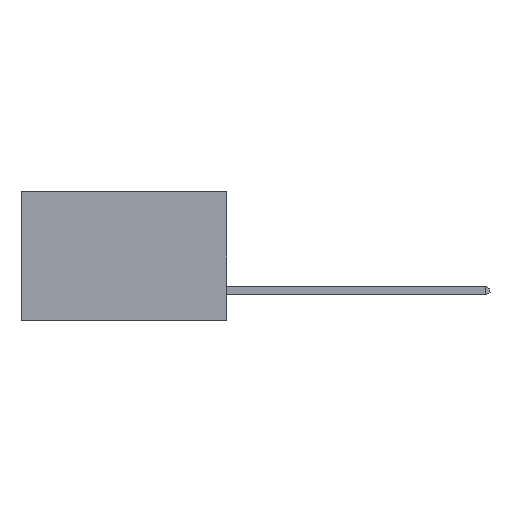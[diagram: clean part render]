
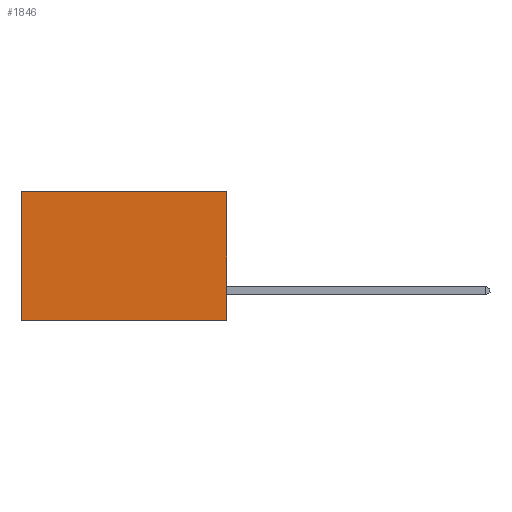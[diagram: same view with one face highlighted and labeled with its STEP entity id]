
A CAD part, left-side view. The second image highlights one B-rep face of the part: STEP entity #1846.
In plain terms, the highlighted planar face has unit normal (-1, 0, 0).
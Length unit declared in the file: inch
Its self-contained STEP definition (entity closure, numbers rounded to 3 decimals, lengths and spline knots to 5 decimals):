
#250 = CARTESIAN_POINT ( 'NONE',  ( 0.277, 0., -0.37 ) ) ;
#343 = DIRECTION ( 'NONE',  ( 1., 0., 0. ) ) ;
#647 = VECTOR ( 'NONE', #4072, 39.37008 ) ;
#1846 = ADVANCED_FACE ( 'NONE', ( #2296 ), #9590, .F. ) ;
#1884 = ORIENTED_EDGE ( 'NONE', *, *, #5309, .T. ) ;
#1910 = ORIENTED_EDGE ( 'NONE', *, *, #5973, .F. ) ;
#1949 = ORIENTED_EDGE ( 'NONE', *, *, #6731, .F. ) ;
#1982 = CARTESIAN_POINT ( 'NONE',  ( 0.277, 0.59, -0.37 ) ) ;
#2050 = ORIENTED_EDGE ( 'NONE', *, *, #12123, .T. ) ;
#2061 = DIRECTION ( 'NONE',  ( 0., 0., -1. ) ) ;
#2296 = FACE_OUTER_BOUND ( 'NONE', #9762, .T. ) ;
#2571 = VECTOR ( 'NONE', #3157, 39.37008 ) ;
#2828 = VERTEX_POINT ( 'NONE', #1982 ) ;
#3022 = CARTESIAN_POINT ( 'NONE',  ( 0.277, 0., 0. ) ) ;
#3157 = DIRECTION ( 'NONE',  ( 0., 0., -1. ) ) ;
#4072 = DIRECTION ( 'NONE',  ( 0., 1., 0. ) ) ;
#5309 = EDGE_CURVE ( 'NONE', #9479, #2828, #12591, .T. ) ;
#5416 = VECTOR ( 'NONE', #11059, 39.37008 ) ;
#5551 = VECTOR ( 'NONE', #2061, 39.37008 ) ;
#5873 = LINE ( 'NONE', #7092, #5551 ) ;
#5973 = EDGE_CURVE ( 'NONE', #10830, #2828, #7963, .T. ) ;
#6114 = LINE ( 'NONE', #3022, #647 ) ;
#6232 = CARTESIAN_POINT ( 'NONE',  ( 0.277, 0., -0.37 ) ) ;
#6429 = VERTEX_POINT ( 'NONE', #9653 ) ;
#6731 = EDGE_CURVE ( 'NONE', #6429, #10830, #5873, .T. ) ;
#7092 = CARTESIAN_POINT ( 'NONE',  ( 0.277, 0., -0.37 ) ) ;
#7963 = LINE ( 'NONE', #9150, #5416 ) ;
#9150 = CARTESIAN_POINT ( 'NONE',  ( 0.277, 0., -0.37 ) ) ;
#9152 = AXIS2_PLACEMENT_3D ( 'NONE', #6232, #343, #9777 ) ;
#9458 = CARTESIAN_POINT ( 'NONE',  ( 0.277, 0.59, 0. ) ) ;
#9479 = VERTEX_POINT ( 'NONE', #9458 ) ;
#9590 = PLANE ( 'NONE',  #9152 ) ;
#9653 = CARTESIAN_POINT ( 'NONE',  ( 0.277, 0., 0. ) ) ;
#9762 = EDGE_LOOP ( 'NONE', ( #1884, #1910, #1949, #2050 ) ) ;
#9777 = DIRECTION ( 'NONE',  ( 0., 0., -1. ) ) ;
#10036 = CARTESIAN_POINT ( 'NONE',  ( 0.277, 0.59, -0.37 ) ) ;
#10830 = VERTEX_POINT ( 'NONE', #250 ) ;
#11059 = DIRECTION ( 'NONE',  ( 0., 1., 0. ) ) ;
#12123 = EDGE_CURVE ( 'NONE', #6429, #9479, #6114, .T. ) ;
#12591 = LINE ( 'NONE', #10036, #2571 ) ;
